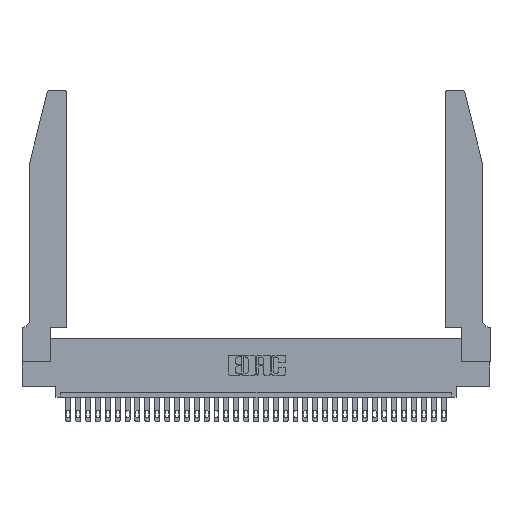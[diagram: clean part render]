
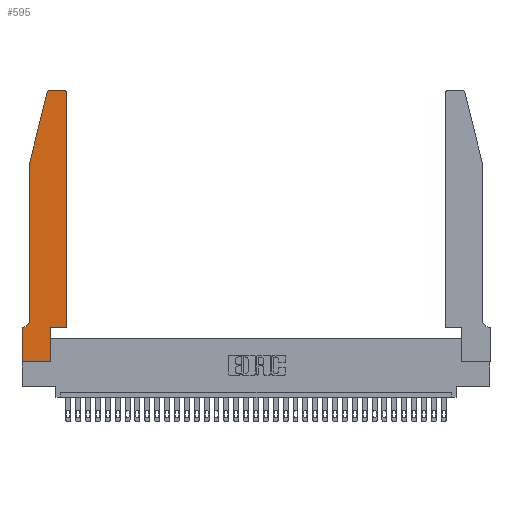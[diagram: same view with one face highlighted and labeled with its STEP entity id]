
A CAD part, top view. The second image highlights one B-rep face of the part: STEP entity #595.
In plain terms, the highlighted planar face has unit normal (0, 0, 1).
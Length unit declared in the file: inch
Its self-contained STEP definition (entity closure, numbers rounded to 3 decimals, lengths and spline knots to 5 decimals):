
#408 = CARTESIAN_POINT ( 'NONE',  ( 0.284, 2.75, 0.37 ) ) ;
#595 = ADVANCED_FACE ( 'NONE', ( #22081 ), #25990, .T. ) ;
#772 = CARTESIAN_POINT ( 'NONE',  ( 0., 0., 0.37 ) ) ;
#862 = VECTOR ( 'NONE', #30489, 39.37008 ) ;
#1416 = VERTEX_POINT ( 'NONE', #27067 ) ;
#1887 = DIRECTION ( 'NONE',  ( 1., 0., 0. ) ) ;
#1898 = EDGE_CURVE ( 'NONE', #2025, #13638, #21177, .T. ) ;
#2016 = VECTOR ( 'NONE', #9422, 39.37008 ) ;
#2025 = VERTEX_POINT ( 'NONE', #22759 ) ;
#2128 = AXIS2_PLACEMENT_3D ( 'NONE', #34122, #9665, #31077 ) ;
#2486 = CARTESIAN_POINT ( 'NONE',  ( 0.0755, 2., 0.37 ) ) ;
#2943 = CARTESIAN_POINT ( 'NONE',  ( 0.0055, 0.35, 0.37 ) ) ;
#3106 = LINE ( 'NONE', #7543, #30716 ) ;
#3223 = VERTEX_POINT ( 'NONE', #772 ) ;
#3293 = CARTESIAN_POINT ( 'NONE',  ( 0.0055, 0.42, 0.37 ) ) ;
#4184 = VECTOR ( 'NONE', #7789, 39.37008 ) ;
#4345 = CARTESIAN_POINT ( 'NONE',  ( 0.4505, 0.35, 0.37 ) ) ;
#4476 = CARTESIAN_POINT ( 'NONE',  ( 0.4205, 2.75, 0.37 ) ) ;
#4578 = VERTEX_POINT ( 'NONE', #408 ) ;
#4995 = CARTESIAN_POINT ( 'NONE',  ( 0.4505, 0.35, 0.37 ) ) ;
#7113 = ORIENTED_EDGE ( 'NONE', *, *, #26241, .T. ) ;
#7349 = ORIENTED_EDGE ( 'NONE', *, *, #11659, .T. ) ;
#7543 = CARTESIAN_POINT ( 'NONE',  ( 0., 0., 0.37 ) ) ;
#7551 = EDGE_CURVE ( 'NONE', #26975, #4578, #8349, .T. ) ;
#7628 = DIRECTION ( 'NONE',  ( 0., 1., 0. ) ) ;
#7789 = DIRECTION ( 'NONE',  ( 1., 0., 0. ) ) ;
#8312 = LINE ( 'NONE', #27960, #14603 ) ;
#8349 = LINE ( 'NONE', #25799, #9673 ) ;
#8369 = DIRECTION ( 'NONE',  ( 0., 0., 1. ) ) ;
#9057 = CARTESIAN_POINT ( 'NONE',  ( 0.0755, 2., 0.37 ) ) ;
#9134 = VERTEX_POINT ( 'NONE', #9599 ) ;
#9418 = EDGE_CURVE ( 'NONE', #17473, #16371, #12024, .T. ) ;
#9422 = DIRECTION ( 'NONE',  ( 0., -1., 0. ) ) ;
#9486 = DIRECTION ( 'NONE',  ( -1., 0., 0. ) ) ;
#9599 = CARTESIAN_POINT ( 'NONE',  ( 0.4505, 2.72, 0.37 ) ) ;
#9665 = DIRECTION ( 'NONE',  ( 0., 0., 1. ) ) ;
#9673 = VECTOR ( 'NONE', #9486, 39.37008 ) ;
#9747 = DIRECTION ( 'NONE',  ( -1., 0., 0. ) ) ;
#10463 = LINE ( 'NONE', #17766, #16248 ) ;
#10719 = DIRECTION ( 'NONE',  ( 1., 0., 0. ) ) ;
#10950 = EDGE_CURVE ( 'NONE', #9134, #26975, #22288, .T. ) ;
#11471 = CARTESIAN_POINT ( 'NONE',  ( 0., 0.35, 0.37 ) ) ;
#11659 = EDGE_CURVE ( 'NONE', #1416, #32827, #21769, .T. ) ;
#12024 = LINE ( 'NONE', #27505, #32550 ) ;
#12721 = AXIS2_PLACEMENT_3D ( 'NONE', #32264, #8369, #10719 ) ;
#13491 = ORIENTED_EDGE ( 'NONE', *, *, #7551, .T. ) ;
#13638 = VERTEX_POINT ( 'NONE', #34227 ) ;
#14110 = ORIENTED_EDGE ( 'NONE', *, *, #16252, .T. ) ;
#14514 = CARTESIAN_POINT ( 'NONE',  ( 0.4205, 2.72, 0.37 ) ) ;
#14537 = DIRECTION ( 'NONE',  ( 0., 1., 0. ) ) ;
#14603 = VECTOR ( 'NONE', #14537, 39.37008 ) ;
#14793 = EDGE_CURVE ( 'NONE', #3223, #33054, #10463, .T. ) ;
#15192 = EDGE_CURVE ( 'NONE', #33054, #2025, #8312, .T. ) ;
#16248 = VECTOR ( 'NONE', #1887, 39.37008 ) ;
#16252 = EDGE_CURVE ( 'NONE', #4578, #17473, #31768, .T. ) ;
#16371 = VERTEX_POINT ( 'NONE', #2486 ) ;
#17225 = DIRECTION ( 'NONE',  ( -0.239, -0.971, 0. ) ) ;
#17473 = VERTEX_POINT ( 'NONE', #34133 ) ;
#17766 = CARTESIAN_POINT ( 'NONE',  ( 0., 0., 0.37 ) ) ;
#18941 = AXIS2_PLACEMENT_3D ( 'NONE', #3293, #27138, #9747 ) ;
#19052 = EDGE_CURVE ( 'NONE', #32827, #31624, #27999, .T. ) ;
#20686 = LINE ( 'NONE', #9057, #2016 ) ;
#20718 = CARTESIAN_POINT ( 'NONE',  ( 0.2865, 0., 0.37 ) ) ;
#20740 = ORIENTED_EDGE ( 'NONE', *, *, #21076, .T. ) ;
#20768 = DIRECTION ( 'NONE',  ( 0., 0., 1. ) ) ;
#20911 = EDGE_LOOP ( 'NONE', ( #13491, #14110, #29837, #20740, #7349, #29154, #7113, #26257, #28403, #34279, #31696, #29891 ) ) ;
#21076 = EDGE_CURVE ( 'NONE', #16371, #1416, #20686, .T. ) ;
#21177 = LINE ( 'NONE', #4345, #4184 ) ;
#21769 = CIRCLE ( 'NONE', #18941, 0.07 ) ;
#22081 = FACE_OUTER_BOUND ( 'NONE', #20911, .T. ) ;
#22280 = VECTOR ( 'NONE', #7628, 39.37008 ) ;
#22288 = CIRCLE ( 'NONE', #29754, 0.03 ) ;
#22759 = CARTESIAN_POINT ( 'NONE',  ( 0.2865, 0.35, 0.37 ) ) ;
#25799 = CARTESIAN_POINT ( 'NONE',  ( 0.2605, 2.75, 0.37 ) ) ;
#25973 = EDGE_CURVE ( 'NONE', #13638, #9134, #29474, .T. ) ;
#25990 = PLANE ( 'NONE',  #2128 ) ;
#26072 = DIRECTION ( 'NONE',  ( 1., 0., 0. ) ) ;
#26241 = EDGE_CURVE ( 'NONE', #31624, #3223, #3106, .T. ) ;
#26257 = ORIENTED_EDGE ( 'NONE', *, *, #14793, .T. ) ;
#26615 = DIRECTION ( 'NONE',  ( 0., -1., 0. ) ) ;
#26975 = VERTEX_POINT ( 'NONE', #4476 ) ;
#27067 = CARTESIAN_POINT ( 'NONE',  ( 0.0755, 0.42, 0.37 ) ) ;
#27138 = DIRECTION ( 'NONE',  ( 0., 0., -1. ) ) ;
#27505 = CARTESIAN_POINT ( 'NONE',  ( 0.0755, 2., 0.37 ) ) ;
#27960 = CARTESIAN_POINT ( 'NONE',  ( 0.2865, 0.35, 0.37 ) ) ;
#27999 = LINE ( 'NONE', #30360, #862 ) ;
#28403 = ORIENTED_EDGE ( 'NONE', *, *, #15192, .T. ) ;
#29154 = ORIENTED_EDGE ( 'NONE', *, *, #19052, .T. ) ;
#29474 = LINE ( 'NONE', #4995, #22280 ) ;
#29754 = AXIS2_PLACEMENT_3D ( 'NONE', #14514, #20768, #26072 ) ;
#29837 = ORIENTED_EDGE ( 'NONE', *, *, #9418, .T. ) ;
#29891 = ORIENTED_EDGE ( 'NONE', *, *, #10950, .T. ) ;
#30360 = CARTESIAN_POINT ( 'NONE',  ( 0.0755, 0.35, 0.37 ) ) ;
#30489 = DIRECTION ( 'NONE',  ( -1., 0., 0. ) ) ;
#30716 = VECTOR ( 'NONE', #26615, 39.37008 ) ;
#31077 = DIRECTION ( 'NONE',  ( 1., 0., 0. ) ) ;
#31624 = VERTEX_POINT ( 'NONE', #11471 ) ;
#31696 = ORIENTED_EDGE ( 'NONE', *, *, #25973, .T. ) ;
#31768 = CIRCLE ( 'NONE', #12721, 0.03 ) ;
#32264 = CARTESIAN_POINT ( 'NONE',  ( 0.284, 2.72, 0.37 ) ) ;
#32550 = VECTOR ( 'NONE', #17225, 39.37008 ) ;
#32827 = VERTEX_POINT ( 'NONE', #2943 ) ;
#33054 = VERTEX_POINT ( 'NONE', #20718 ) ;
#34122 = CARTESIAN_POINT ( 'NONE',  ( 0., 0.35, 0.37 ) ) ;
#34133 = CARTESIAN_POINT ( 'NONE',  ( 0.25487, 2.72718, 0.37 ) ) ;
#34227 = CARTESIAN_POINT ( 'NONE',  ( 0.4505, 0.35, 0.37 ) ) ;
#34279 = ORIENTED_EDGE ( 'NONE', *, *, #1898, .T. ) ;
